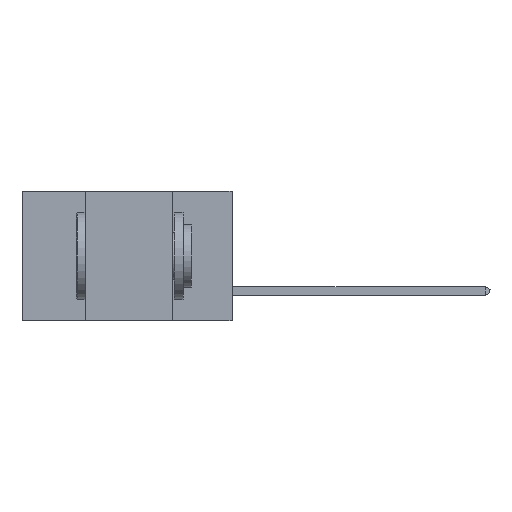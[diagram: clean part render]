
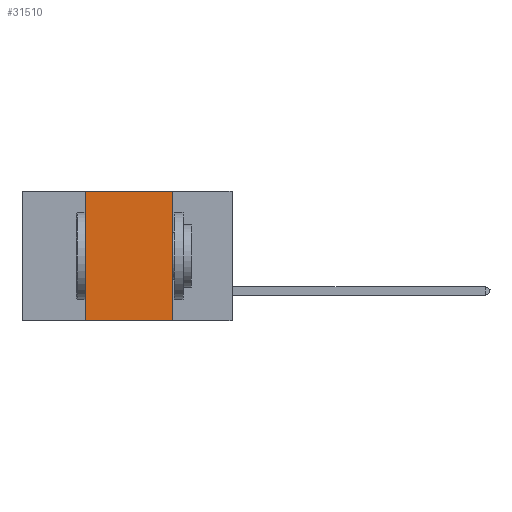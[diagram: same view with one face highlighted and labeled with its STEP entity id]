
A CAD part, left-side view. The second image highlights one B-rep face of the part: STEP entity #31510.
In plain terms, the highlighted planar face has unit normal (-1, 0, 0).
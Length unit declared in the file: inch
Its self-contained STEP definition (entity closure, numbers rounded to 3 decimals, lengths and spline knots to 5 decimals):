
#163 = VECTOR ( 'NONE', #10854, 39.37008 ) ;
#627 = DIRECTION ( 'NONE',  ( 1., 0., 0. ) ) ;
#862 = CARTESIAN_POINT ( 'NONE',  ( 0., 0.6, 0. ) ) ;
#1204 = CARTESIAN_POINT ( 'NONE',  ( 0., 0.17, -0.37 ) ) ;
#1629 = FACE_OUTER_BOUND ( 'NONE', #29768, .T. ) ;
#2581 = VECTOR ( 'NONE', #24920, 39.37008 ) ;
#3428 = ORIENTED_EDGE ( 'NONE', *, *, #33410, .F. ) ;
#7547 = CARTESIAN_POINT ( 'NONE',  ( 0., 0.6, -0.37 ) ) ;
#10854 = DIRECTION ( 'NONE',  ( 0., -1., 0. ) ) ;
#12201 = VERTEX_POINT ( 'NONE', #1204 ) ;
#15242 = LINE ( 'NONE', #31141, #16517 ) ;
#15249 = DIRECTION ( 'NONE',  ( 0., 0., 1. ) ) ;
#15915 = VERTEX_POINT ( 'NONE', #24564 ) ;
#15986 = EDGE_CURVE ( 'NONE', #34898, #15915, #15242, .T. ) ;
#16517 = VECTOR ( 'NONE', #15249, 39.37008 ) ;
#16703 = CARTESIAN_POINT ( 'NONE',  ( 0., 0.6, 0. ) ) ;
#16962 = LINE ( 'NONE', #26528, #26122 ) ;
#17271 = CARTESIAN_POINT ( 'NONE',  ( 0., 0.17, 0. ) ) ;
#18256 = LINE ( 'NONE', #7547, #2581 ) ;
#19001 = CARTESIAN_POINT ( 'NONE',  ( 0., 0.42, -0.37 ) ) ;
#20213 = ORIENTED_EDGE ( 'NONE', *, *, #20905, .F. ) ;
#20527 = DIRECTION ( 'NONE',  ( 0., 0., -1. ) ) ;
#20905 = EDGE_CURVE ( 'NONE', #27772, #12201, #16962, .T. ) ;
#21046 = DIRECTION ( 'NONE',  ( 0., 0., -1. ) ) ;
#22305 = AXIS2_PLACEMENT_3D ( 'NONE', #862, #627, #20527 ) ;
#24564 = CARTESIAN_POINT ( 'NONE',  ( 0., 0.42, 0. ) ) ;
#24831 = ORIENTED_EDGE ( 'NONE', *, *, #29960, .T. ) ;
#24920 = DIRECTION ( 'NONE',  ( 0., -1., 0. ) ) ;
#25896 = PLANE ( 'NONE',  #22305 ) ;
#26122 = VECTOR ( 'NONE', #21046, 39.37008 ) ;
#26528 = CARTESIAN_POINT ( 'NONE',  ( 0., 0.17, 0. ) ) ;
#27772 = VERTEX_POINT ( 'NONE', #17271 ) ;
#28422 = LINE ( 'NONE', #16703, #163 ) ;
#29768 = EDGE_LOOP ( 'NONE', ( #20213, #3428, #35362, #24831 ) ) ;
#29960 = EDGE_CURVE ( 'NONE', #34898, #12201, #18256, .T. ) ;
#31141 = CARTESIAN_POINT ( 'NONE',  ( 0., 0.42, 0. ) ) ;
#31510 = ADVANCED_FACE ( 'NONE', ( #1629 ), #25896, .F. ) ;
#33410 = EDGE_CURVE ( 'NONE', #15915, #27772, #28422, .T. ) ;
#34898 = VERTEX_POINT ( 'NONE', #19001 ) ;
#35362 = ORIENTED_EDGE ( 'NONE', *, *, #15986, .F. ) ;
